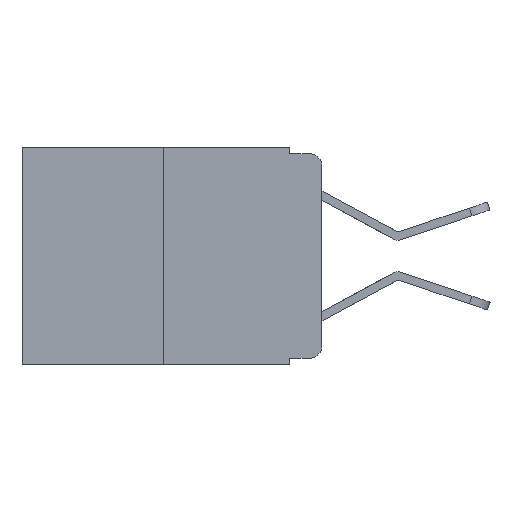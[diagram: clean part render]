
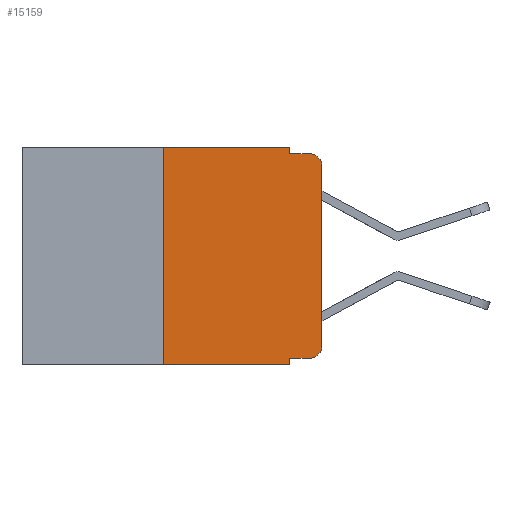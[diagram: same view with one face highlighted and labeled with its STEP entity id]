
A CAD part, left-side view. The second image highlights one B-rep face of the part: STEP entity #15159.
In plain terms, the highlighted planar face has unit normal (-1, 0, 0).
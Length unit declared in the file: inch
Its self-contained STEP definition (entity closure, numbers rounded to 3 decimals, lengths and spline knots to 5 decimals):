
#525 = VERTEX_POINT ( 'NONE', #10989 ) ;
#564 = DIRECTION ( 'NONE',  ( 0., 0., 1. ) ) ;
#839 = LINE ( 'NONE', #9550, #8598 ) ;
#979 = CARTESIAN_POINT ( 'NONE',  ( 0., 0.051, -0.01 ) ) ;
#1166 = EDGE_CURVE ( 'NONE', #15118, #4088, #11544, .T. ) ;
#1242 = CARTESIAN_POINT ( 'NONE',  ( 0., 0.051, -0.333 ) ) ;
#1783 = LINE ( 'NONE', #8729, #11578 ) ;
#1791 = CARTESIAN_POINT ( 'NONE',  ( 0., 0.25, 0. ) ) ;
#1844 = VECTOR ( 'NONE', #8026, 39.37008 ) ;
#1854 = DIRECTION ( 'NONE',  ( 0., 0., -1. ) ) ;
#2232 = DIRECTION ( 'NONE',  ( 0., -1., 0. ) ) ;
#2300 = VECTOR ( 'NONE', #7691, 39.37008 ) ;
#2312 = VECTOR ( 'NONE', #564, 39.37008 ) ;
#2368 = VERTEX_POINT ( 'NONE', #10567 ) ;
#2370 = CIRCLE ( 'NONE', #10901, 0.02 ) ;
#2453 = LINE ( 'NONE', #6253, #15047 ) ;
#2515 = ORIENTED_EDGE ( 'NONE', *, *, #9896, .F. ) ;
#2518 = VERTEX_POINT ( 'NONE', #1242 ) ;
#2524 = ORIENTED_EDGE ( 'NONE', *, *, #11478, .F. ) ;
#2767 = VECTOR ( 'NONE', #5295, 39.37008 ) ;
#3353 = CARTESIAN_POINT ( 'NONE',  ( 0., 0.25, 0. ) ) ;
#3522 = CARTESIAN_POINT ( 'NONE',  ( 0., 0.473, 0. ) ) ;
#3578 = PLANE ( 'NONE',  #11184 ) ;
#3707 = ORIENTED_EDGE ( 'NONE', *, *, #12614, .T. ) ;
#3922 = CARTESIAN_POINT ( 'NONE',  ( 0., 0.051, -0.01 ) ) ;
#3950 = ORIENTED_EDGE ( 'NONE', *, *, #1166, .T. ) ;
#4088 = VERTEX_POINT ( 'NONE', #9149 ) ;
#4536 = CARTESIAN_POINT ( 'NONE',  ( 0., 0., -0.313 ) ) ;
#4707 = ORIENTED_EDGE ( 'NONE', *, *, #8346, .T. ) ;
#5295 = DIRECTION ( 'NONE',  ( 0., 0., -1. ) ) ;
#5350 = LINE ( 'NONE', #979, #1844 ) ;
#5541 = VERTEX_POINT ( 'NONE', #12285 ) ;
#5832 = DIRECTION ( 'NONE',  ( 0., -1., 0. ) ) ;
#6253 = CARTESIAN_POINT ( 'NONE',  ( 0., 0.473, -0.343 ) ) ;
#6451 = ORIENTED_EDGE ( 'NONE', *, *, #10570, .F. ) ;
#6579 = CARTESIAN_POINT ( 'NONE',  ( 0., 0.051, -0.343 ) ) ;
#6889 = ORIENTED_EDGE ( 'NONE', *, *, #14308, .F. ) ;
#6982 = CARTESIAN_POINT ( 'NONE',  ( 0., 0.02, -0.313 ) ) ;
#7128 = AXIS2_PLACEMENT_3D ( 'NONE', #12007, #13563, #10793 ) ;
#7634 = EDGE_CURVE ( 'NONE', #8724, #2368, #5350, .T. ) ;
#7691 = DIRECTION ( 'NONE',  ( 0., 0., 1. ) ) ;
#7779 = ORIENTED_EDGE ( 'NONE', *, *, #9139, .T. ) ;
#8026 = DIRECTION ( 'NONE',  ( 0., -1., 0. ) ) ;
#8170 = DIRECTION ( 'NONE',  ( 0., 0., -1. ) ) ;
#8346 = EDGE_CURVE ( 'NONE', #5541, #15118, #2370, .T. ) ;
#8534 = EDGE_LOOP ( 'NONE', ( #3950, #7779, #9159, #6889, #6451, #2524, #3707, #2515, #9229, #4707 ) ) ;
#8598 = VECTOR ( 'NONE', #5832, 39.37008 ) ;
#8724 = VERTEX_POINT ( 'NONE', #3922 ) ;
#8729 = CARTESIAN_POINT ( 'NONE',  ( 0., 0.051, 0. ) ) ;
#8928 = VECTOR ( 'NONE', #2232, 39.37008 ) ;
#9139 = EDGE_CURVE ( 'NONE', #4088, #2368, #13099, .T. ) ;
#9149 = CARTESIAN_POINT ( 'NONE',  ( 0., 0., -0.03 ) ) ;
#9159 = ORIENTED_EDGE ( 'NONE', *, *, #7634, .F. ) ;
#9229 = ORIENTED_EDGE ( 'NONE', *, *, #12318, .T. ) ;
#9256 = DIRECTION ( 'NONE',  ( -1., 0., 0. ) ) ;
#9550 = CARTESIAN_POINT ( 'NONE',  ( 0., 0.473, 0. ) ) ;
#9863 = DIRECTION ( 'NONE',  ( 0., -1., 0. ) ) ;
#9896 = EDGE_CURVE ( 'NONE', #2518, #10082, #1783, .T. ) ;
#10082 = VERTEX_POINT ( 'NONE', #6579 ) ;
#10567 = CARTESIAN_POINT ( 'NONE',  ( 0., 0.02, -0.01 ) ) ;
#10570 = EDGE_CURVE ( 'NONE', #11059, #10666, #839, .T. ) ;
#10666 = VERTEX_POINT ( 'NONE', #13356 ) ;
#10793 = DIRECTION ( 'NONE',  ( 0., 0., -1. ) ) ;
#10901 = AXIS2_PLACEMENT_3D ( 'NONE', #6982, #9256, #8170 ) ;
#10989 = CARTESIAN_POINT ( 'NONE',  ( 0., 0.25, -0.343 ) ) ;
#11059 = VERTEX_POINT ( 'NONE', #3353 ) ;
#11151 = LINE ( 'NONE', #14077, #8928 ) ;
#11184 = AXIS2_PLACEMENT_3D ( 'NONE', #3522, #15214, #11795 ) ;
#11478 = EDGE_CURVE ( 'NONE', #525, #11059, #11751, .T. ) ;
#11544 = LINE ( 'NONE', #13616, #2300 ) ;
#11578 = VECTOR ( 'NONE', #1854, 39.37008 ) ;
#11646 = LINE ( 'NONE', #14680, #2767 ) ;
#11751 = LINE ( 'NONE', #1791, #2312 ) ;
#11795 = DIRECTION ( 'NONE',  ( 0., 0., -1. ) ) ;
#12007 = CARTESIAN_POINT ( 'NONE',  ( 0., 0.02, -0.03 ) ) ;
#12285 = CARTESIAN_POINT ( 'NONE',  ( 0., 0.02, -0.333 ) ) ;
#12318 = EDGE_CURVE ( 'NONE', #2518, #5541, #11151, .T. ) ;
#12364 = FACE_OUTER_BOUND ( 'NONE', #8534, .T. ) ;
#12614 = EDGE_CURVE ( 'NONE', #525, #10082, #2453, .T. ) ;
#13099 = CIRCLE ( 'NONE', #7128, 0.02 ) ;
#13356 = CARTESIAN_POINT ( 'NONE',  ( 0., 0.051, 0. ) ) ;
#13563 = DIRECTION ( 'NONE',  ( -1., 0., 0. ) ) ;
#13616 = CARTESIAN_POINT ( 'NONE',  ( 0., 0., 0. ) ) ;
#14077 = CARTESIAN_POINT ( 'NONE',  ( 0., 0.051, -0.333 ) ) ;
#14308 = EDGE_CURVE ( 'NONE', #10666, #8724, #11646, .T. ) ;
#14680 = CARTESIAN_POINT ( 'NONE',  ( 0., 0.051, 0. ) ) ;
#15047 = VECTOR ( 'NONE', #9863, 39.37008 ) ;
#15118 = VERTEX_POINT ( 'NONE', #4536 ) ;
#15159 = ADVANCED_FACE ( 'NONE', ( #12364 ), #3578, .F. ) ;
#15214 = DIRECTION ( 'NONE',  ( 1., 0., 0. ) ) ;
